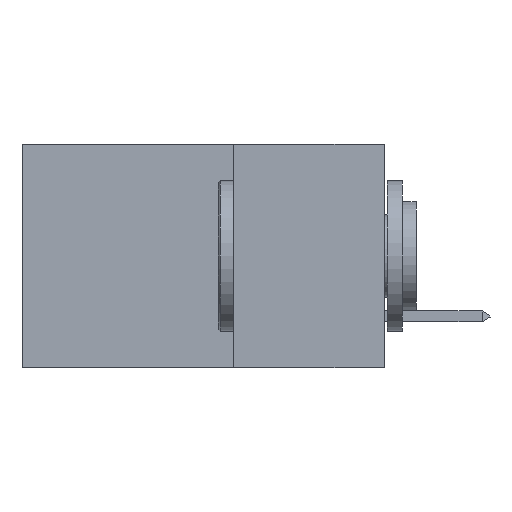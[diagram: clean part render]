
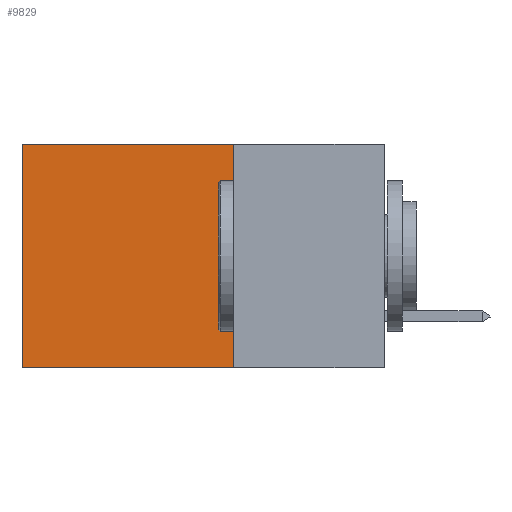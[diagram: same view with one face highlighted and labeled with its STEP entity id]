
A CAD part, left-side view. The second image highlights one B-rep face of the part: STEP entity #9829.
In plain terms, the highlighted planar face has unit normal (-1, 0, 0).
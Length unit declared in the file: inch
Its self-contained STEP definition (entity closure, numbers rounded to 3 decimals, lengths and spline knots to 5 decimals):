
#487 = VECTOR ( 'NONE', #7549, 39.37008 ) ;
#496 = VECTOR ( 'NONE', #3431, 39.37008 ) ;
#965 = ORIENTED_EDGE ( 'NONE', *, *, #9600, .T. ) ;
#1173 = PLANE ( 'NONE',  #9803 ) ;
#2084 = LINE ( 'NONE', #15121, #5292 ) ;
#2656 = CARTESIAN_POINT ( 'NONE',  ( 0.2875, 0.6, -0.37 ) ) ;
#3431 = DIRECTION ( 'NONE',  ( 0., 1., 0. ) ) ;
#3719 = LINE ( 'NONE', #17618, #487 ) ;
#4201 = LINE ( 'NONE', #16159, #10491 ) ;
#4596 = EDGE_CURVE ( 'NONE', #8990, #7381, #4201, .T. ) ;
#4954 = DIRECTION ( 'NONE',  ( 0., 0., -1. ) ) ;
#5058 = CARTESIAN_POINT ( 'NONE',  ( 0.2875, 0.25, 0. ) ) ;
#5292 = VECTOR ( 'NONE', #6087, 39.37008 ) ;
#5423 = VERTEX_POINT ( 'NONE', #16974 ) ;
#6087 = DIRECTION ( 'NONE',  ( 0., 0., -1. ) ) ;
#6595 = VERTEX_POINT ( 'NONE', #2656 ) ;
#7381 = VERTEX_POINT ( 'NONE', #8182 ) ;
#7549 = DIRECTION ( 'NONE',  ( 0., 0., -1. ) ) ;
#7572 = DIRECTION ( 'NONE',  ( 0., 1., 0. ) ) ;
#8182 = CARTESIAN_POINT ( 'NONE',  ( 0.2875, 0.6, 0. ) ) ;
#8967 = EDGE_LOOP ( 'NONE', ( #965, #12647, #9228, #15171 ) ) ;
#8990 = VERTEX_POINT ( 'NONE', #5058 ) ;
#9228 = ORIENTED_EDGE ( 'NONE', *, *, #10054, .F. ) ;
#9600 = EDGE_CURVE ( 'NONE', #7381, #6595, #2084, .T. ) ;
#9803 = AXIS2_PLACEMENT_3D ( 'NONE', #17298, #13211, #4954 ) ;
#9829 = ADVANCED_FACE ( 'NONE', ( #16818 ), #1173, .F. ) ;
#10054 = EDGE_CURVE ( 'NONE', #8990, #5423, #3719, .T. ) ;
#10479 = CARTESIAN_POINT ( 'NONE',  ( 0.2875, 0.25, -0.37 ) ) ;
#10491 = VECTOR ( 'NONE', #7572, 39.37008 ) ;
#12647 = ORIENTED_EDGE ( 'NONE', *, *, #18702, .F. ) ;
#13211 = DIRECTION ( 'NONE',  ( 1., 0., 0. ) ) ;
#15121 = CARTESIAN_POINT ( 'NONE',  ( 0.2875, 0.6, 0. ) ) ;
#15171 = ORIENTED_EDGE ( 'NONE', *, *, #4596, .T. ) ;
#16159 = CARTESIAN_POINT ( 'NONE',  ( 0.2875, 0.25, 0. ) ) ;
#16363 = LINE ( 'NONE', #10479, #496 ) ;
#16818 = FACE_OUTER_BOUND ( 'NONE', #8967, .T. ) ;
#16974 = CARTESIAN_POINT ( 'NONE',  ( 0.2875, 0.25, -0.37 ) ) ;
#17298 = CARTESIAN_POINT ( 'NONE',  ( 0.2875, 0.25, 0. ) ) ;
#17618 = CARTESIAN_POINT ( 'NONE',  ( 0.2875, 0.25, 0. ) ) ;
#18702 = EDGE_CURVE ( 'NONE', #5423, #6595, #16363, .T. ) ;
